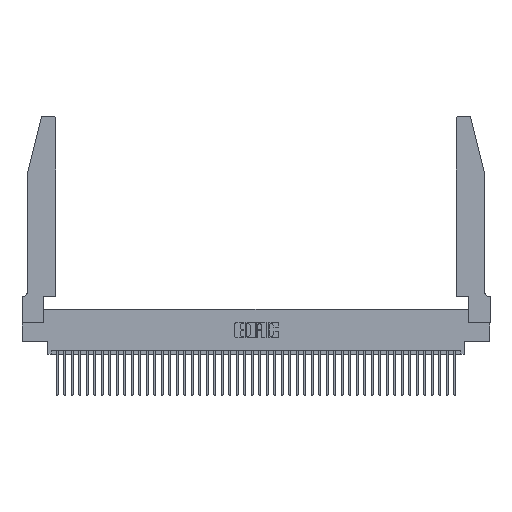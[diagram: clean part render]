
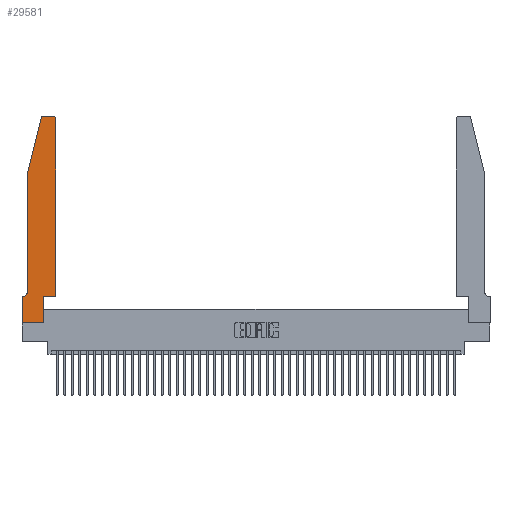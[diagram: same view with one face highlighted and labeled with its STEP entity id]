
A CAD part, top view. The second image highlights one B-rep face of the part: STEP entity #29581.
In plain terms, the highlighted planar face has unit normal (0, 0, 1).
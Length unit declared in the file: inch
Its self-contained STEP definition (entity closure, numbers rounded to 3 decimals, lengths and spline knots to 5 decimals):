
#632 = CIRCLE ( 'NONE', #12883, 0.03 ) ;
#756 = VERTEX_POINT ( 'NONE', #7276 ) ;
#1400 = VECTOR ( 'NONE', #17553, 39.37008 ) ;
#2424 = EDGE_CURVE ( 'NONE', #17573, #18030, #18795, .T. ) ;
#2737 = DIRECTION ( 'NONE',  ( 0., 0., 1. ) ) ;
#4733 = FACE_OUTER_BOUND ( 'NONE', #19199, .T. ) ;
#5211 = CARTESIAN_POINT ( 'NONE',  ( 0.0755, 2., 0.37 ) ) ;
#6059 = ORIENTED_EDGE ( 'NONE', *, *, #33974, .T. ) ;
#6225 = CARTESIAN_POINT ( 'NONE',  ( 0., 0., 0.37 ) ) ;
#6476 = CARTESIAN_POINT ( 'NONE',  ( 0.4205, 2.72, 0.37 ) ) ;
#6689 = CARTESIAN_POINT ( 'NONE',  ( 0.2605, 2.75, 0.37 ) ) ;
#7093 = LINE ( 'NONE', #37681, #27072 ) ;
#7183 = CARTESIAN_POINT ( 'NONE',  ( 0.4505, 2.72, 0.37 ) ) ;
#7276 = CARTESIAN_POINT ( 'NONE',  ( 0.4505, 0.35, 0.37 ) ) ;
#7748 = VECTOR ( 'NONE', #7822, 39.37008 ) ;
#7822 = DIRECTION ( 'NONE',  ( -1., 0., 0. ) ) ;
#9315 = VECTOR ( 'NONE', #38347, 39.37008 ) ;
#9648 = CARTESIAN_POINT ( 'NONE',  ( 0.4505, 0.35, 0.37 ) ) ;
#9814 = LINE ( 'NONE', #6225, #27474 ) ;
#9928 = DIRECTION ( 'NONE',  ( 1., 0., 0. ) ) ;
#10140 = PLANE ( 'NONE',  #15212 ) ;
#10182 = DIRECTION ( 'NONE',  ( 1., 0., 0. ) ) ;
#10735 = VERTEX_POINT ( 'NONE', #20970 ) ;
#11659 = ORIENTED_EDGE ( 'NONE', *, *, #17994, .T. ) ;
#11688 = EDGE_CURVE ( 'NONE', #20691, #17659, #40827, .T. ) ;
#11762 = VERTEX_POINT ( 'NONE', #33200 ) ;
#12275 = DIRECTION ( 'NONE',  ( 0., 0., -1. ) ) ;
#12789 = VECTOR ( 'NONE', #33472, 39.37008 ) ;
#12883 = AXIS2_PLACEMENT_3D ( 'NONE', #6476, #31213, #10182 ) ;
#13280 = DIRECTION ( 'NONE',  ( 1., 0., 0. ) ) ;
#13307 = DIRECTION ( 'NONE',  ( 0., 1., 0. ) ) ;
#13351 = CIRCLE ( 'NONE', #27194, 0.07 ) ;
#13438 = VERTEX_POINT ( 'NONE', #35845 ) ;
#13575 = ORIENTED_EDGE ( 'NONE', *, *, #15274, .T. ) ;
#13743 = DIRECTION ( 'NONE',  ( 0., 0., 1. ) ) ;
#14124 = VERTEX_POINT ( 'NONE', #18170 ) ;
#14142 = VECTOR ( 'NONE', #42877, 39.37008 ) ;
#15212 = AXIS2_PLACEMENT_3D ( 'NONE', #37978, #13743, #38127 ) ;
#15274 = EDGE_CURVE ( 'NONE', #11762, #756, #28362, .T. ) ;
#15538 = ORIENTED_EDGE ( 'NONE', *, *, #34542, .T. ) ;
#17267 = ORIENTED_EDGE ( 'NONE', *, *, #28717, .T. ) ;
#17553 = DIRECTION ( 'NONE',  ( 0., 1., 0. ) ) ;
#17573 = VERTEX_POINT ( 'NONE', #25238 ) ;
#17659 = VERTEX_POINT ( 'NONE', #25698 ) ;
#17994 = EDGE_CURVE ( 'NONE', #756, #28454, #19459, .T. ) ;
#18030 = VERTEX_POINT ( 'NONE', #31559 ) ;
#18170 = CARTESIAN_POINT ( 'NONE',  ( 0.0055, 0.35, 0.37 ) ) ;
#18393 = LINE ( 'NONE', #42739, #7748 ) ;
#18795 = LINE ( 'NONE', #6689, #9315 ) ;
#19103 = CIRCLE ( 'NONE', #34662, 0.03 ) ;
#19199 = EDGE_LOOP ( 'NONE', ( #29333, #21868, #35275, #15538, #17267, #6059, #20902, #35324, #42325, #13575, #11659, #41986 ) ) ;
#19459 = LINE ( 'NONE', #41843, #1400 ) ;
#20053 = EDGE_CURVE ( 'NONE', #28454, #17573, #632, .T. ) ;
#20691 = VERTEX_POINT ( 'NONE', #41147 ) ;
#20902 = ORIENTED_EDGE ( 'NONE', *, *, #11688, .T. ) ;
#20970 = CARTESIAN_POINT ( 'NONE',  ( 0.0755, 2., 0.37 ) ) ;
#21868 = ORIENTED_EDGE ( 'NONE', *, *, #26605, .T. ) ;
#22148 = CARTESIAN_POINT ( 'NONE',  ( 0., 0., 0.37 ) ) ;
#24204 = CARTESIAN_POINT ( 'NONE',  ( 0.284, 2.72, 0.37 ) ) ;
#25238 = CARTESIAN_POINT ( 'NONE',  ( 0.4205, 2.75, 0.37 ) ) ;
#25698 = CARTESIAN_POINT ( 'NONE',  ( 0., 0., 0.37 ) ) ;
#26112 = VERTEX_POINT ( 'NONE', #30313 ) ;
#26605 = EDGE_CURVE ( 'NONE', #18030, #36494, #19103, .T. ) ;
#27072 = VECTOR ( 'NONE', #13307, 39.37008 ) ;
#27194 = AXIS2_PLACEMENT_3D ( 'NONE', #33224, #12275, #36690 ) ;
#27474 = VECTOR ( 'NONE', #9928, 39.37008 ) ;
#27687 = DIRECTION ( 'NONE',  ( 1., 0., 0. ) ) ;
#28362 = LINE ( 'NONE', #9648, #45678 ) ;
#28454 = VERTEX_POINT ( 'NONE', #7183 ) ;
#28717 = EDGE_CURVE ( 'NONE', #13438, #14124, #13351, .T. ) ;
#29333 = ORIENTED_EDGE ( 'NONE', *, *, #2424, .T. ) ;
#29581 = ADVANCED_FACE ( 'NONE', ( #4733 ), #10140, .T. ) ;
#30033 = CARTESIAN_POINT ( 'NONE',  ( 0.25487, 2.72718, 0.37 ) ) ;
#30185 = EDGE_CURVE ( 'NONE', #17659, #26112, #9814, .T. ) ;
#30313 = CARTESIAN_POINT ( 'NONE',  ( 0.2865, 0., 0.37 ) ) ;
#31213 = DIRECTION ( 'NONE',  ( 0., 0., 1. ) ) ;
#31559 = CARTESIAN_POINT ( 'NONE',  ( 0.284, 2.75, 0.37 ) ) ;
#33200 = CARTESIAN_POINT ( 'NONE',  ( 0.2865, 0.35, 0.37 ) ) ;
#33224 = CARTESIAN_POINT ( 'NONE',  ( 0.0055, 0.42, 0.37 ) ) ;
#33472 = DIRECTION ( 'NONE',  ( 0., -1., 0. ) ) ;
#33614 = EDGE_CURVE ( 'NONE', #36494, #10735, #44434, .T. ) ;
#33662 = VECTOR ( 'NONE', #33990, 39.37008 ) ;
#33974 = EDGE_CURVE ( 'NONE', #14124, #20691, #18393, .T. ) ;
#33990 = DIRECTION ( 'NONE',  ( -0.239, -0.971, 0. ) ) ;
#34542 = EDGE_CURVE ( 'NONE', #10735, #13438, #41692, .T. ) ;
#34662 = AXIS2_PLACEMENT_3D ( 'NONE', #24204, #2737, #27687 ) ;
#34727 = EDGE_CURVE ( 'NONE', #26112, #11762, #7093, .T. ) ;
#35275 = ORIENTED_EDGE ( 'NONE', *, *, #33614, .T. ) ;
#35324 = ORIENTED_EDGE ( 'NONE', *, *, #30185, .T. ) ;
#35845 = CARTESIAN_POINT ( 'NONE',  ( 0.0755, 0.42, 0.37 ) ) ;
#36494 = VERTEX_POINT ( 'NONE', #30033 ) ;
#36690 = DIRECTION ( 'NONE',  ( -1., 0., 0. ) ) ;
#37468 = CARTESIAN_POINT ( 'NONE',  ( 0.0755, 2., 0.37 ) ) ;
#37681 = CARTESIAN_POINT ( 'NONE',  ( 0.2865, 0.35, 0.37 ) ) ;
#37978 = CARTESIAN_POINT ( 'NONE',  ( 0., 0.35, 0.37 ) ) ;
#38127 = DIRECTION ( 'NONE',  ( 1., 0., 0. ) ) ;
#38347 = DIRECTION ( 'NONE',  ( -1., 0., 0. ) ) ;
#40827 = LINE ( 'NONE', #22148, #14142 ) ;
#41147 = CARTESIAN_POINT ( 'NONE',  ( 0., 0.35, 0.37 ) ) ;
#41692 = LINE ( 'NONE', #5211, #12789 ) ;
#41843 = CARTESIAN_POINT ( 'NONE',  ( 0.4505, 0.35, 0.37 ) ) ;
#41986 = ORIENTED_EDGE ( 'NONE', *, *, #20053, .T. ) ;
#42325 = ORIENTED_EDGE ( 'NONE', *, *, #34727, .T. ) ;
#42739 = CARTESIAN_POINT ( 'NONE',  ( 0.0755, 0.35, 0.37 ) ) ;
#42877 = DIRECTION ( 'NONE',  ( 0., -1., 0. ) ) ;
#44434 = LINE ( 'NONE', #37468, #33662 ) ;
#45678 = VECTOR ( 'NONE', #13280, 39.37008 ) ;
